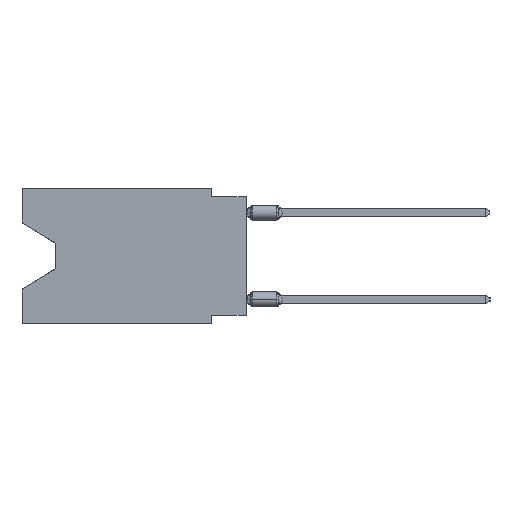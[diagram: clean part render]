
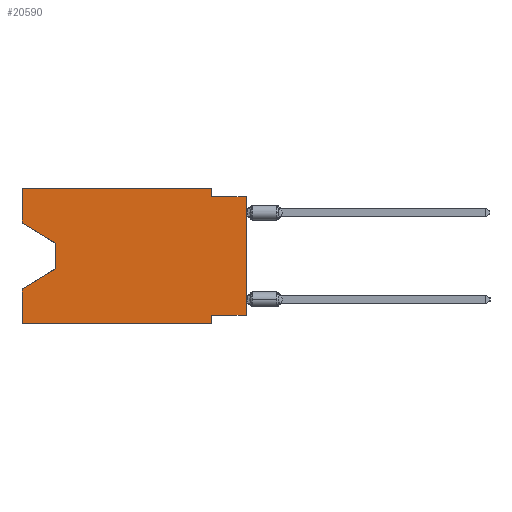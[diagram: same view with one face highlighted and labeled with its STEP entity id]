
A CAD part, left-side view. The second image highlights one B-rep face of the part: STEP entity #20590.
In plain terms, the highlighted planar face has unit normal (-1, 0, 0).
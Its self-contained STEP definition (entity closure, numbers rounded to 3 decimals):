
#54 = ORIENTED_EDGE ( 'NONE', *, *, #9145, .F. ) ;
#492 = AXIS2_PLACEMENT_3D ( 'NONE', #55331, #2793, #37650 ) ;
#593 = CARTESIAN_POINT ( 'NONE',  ( 0., 16.383, 0. ) ) ;
#1018 = EDGE_LOOP ( 'NONE', ( #4741, #35743, #3270, #43502, #29991, #54, #26393, #41804, #6170, #9267, #16644, #18646 ) ) ;
#1906 = VECTOR ( 'NONE', #36949, 1000. ) ;
#2367 = LINE ( 'NONE', #6391, #1906 ) ;
#2661 = EDGE_CURVE ( 'NONE', #33258, #40335, #24436, .T. ) ;
#2711 = CARTESIAN_POINT ( 'NONE',  ( 0., 16.383, 0. ) ) ;
#2793 = DIRECTION ( 'NONE',  ( 1., 0., 0. ) ) ;
#2820 = LINE ( 'NONE', #47371, #49563 ) ;
#3062 = EDGE_CURVE ( 'NONE', #53417, #13756, #2367, .T. ) ;
#3233 = VECTOR ( 'NONE', #11815, 1000. ) ;
#3270 = ORIENTED_EDGE ( 'NONE', *, *, #39068, .T. ) ;
#3426 = EDGE_CURVE ( 'NONE', #18041, #45222, #9479, .T. ) ;
#3548 = EDGE_CURVE ( 'NONE', #38810, #24985, #23474, .T. ) ;
#3928 = CARTESIAN_POINT ( 'NONE',  ( 0., 2.54, 0. ) ) ;
#4708 = CARTESIAN_POINT ( 'NONE',  ( 0., 13.97, -4.013 ) ) ;
#4741 = ORIENTED_EDGE ( 'NONE', *, *, #3548, .T. ) ;
#5100 = CARTESIAN_POINT ( 'NONE',  ( 0., 2.54, -9.906 ) ) ;
#6170 = ORIENTED_EDGE ( 'NONE', *, *, #18437, .F. ) ;
#6234 = CARTESIAN_POINT ( 'NONE',  ( 0., 13.97, -4.013 ) ) ;
#6391 = CARTESIAN_POINT ( 'NONE',  ( 0., 16.383, 0. ) ) ;
#6787 = VERTEX_POINT ( 'NONE', #23119 ) ;
#7640 = LINE ( 'NONE', #3928, #50952 ) ;
#9145 = EDGE_CURVE ( 'NONE', #18328, #13405, #28743, .T. ) ;
#9267 = ORIENTED_EDGE ( 'NONE', *, *, #42584, .F. ) ;
#9479 = LINE ( 'NONE', #26908, #35715 ) ;
#10612 = CARTESIAN_POINT ( 'NONE',  ( 0., 16.383, -2.546 ) ) ;
#10644 = CARTESIAN_POINT ( 'NONE',  ( 0., 2.54, 0. ) ) ;
#10819 = LINE ( 'NONE', #37380, #25836 ) ;
#11815 = DIRECTION ( 'NONE',  ( 0., 0.855, -0.519 ) ) ;
#12222 = FACE_OUTER_BOUND ( 'NONE', #1018, .T. ) ;
#12529 = EDGE_CURVE ( 'NONE', #53417, #13405, #22379, .T. ) ;
#12964 = CARTESIAN_POINT ( 'NONE',  ( 0., 16.383, -9.906 ) ) ;
#13405 = VERTEX_POINT ( 'NONE', #5100 ) ;
#13478 = EDGE_CURVE ( 'NONE', #24985, #6787, #27385, .T. ) ;
#13518 = DIRECTION ( 'NONE',  ( 0., -1., 0. ) ) ;
#13756 = VERTEX_POINT ( 'NONE', #19018 ) ;
#14717 = VECTOR ( 'NONE', #40891, 1000. ) ;
#16524 = VECTOR ( 'NONE', #36237, 1000. ) ;
#16644 = ORIENTED_EDGE ( 'NONE', *, *, #2661, .F. ) ;
#17366 = VECTOR ( 'NONE', #20144, 1000. ) ;
#18041 = VERTEX_POINT ( 'NONE', #33754 ) ;
#18328 = VERTEX_POINT ( 'NONE', #49402 ) ;
#18437 = EDGE_CURVE ( 'NONE', #20125, #45222, #2820, .T. ) ;
#18609 = CARTESIAN_POINT ( 'NONE',  ( 0., 2.54, -0.635 ) ) ;
#18646 = ORIENTED_EDGE ( 'NONE', *, *, #19426, .F. ) ;
#19018 = CARTESIAN_POINT ( 'NONE',  ( 0., 16.383, -7.36 ) ) ;
#19426 = EDGE_CURVE ( 'NONE', #38810, #33258, #48273, .T. ) ;
#20125 = VERTEX_POINT ( 'NONE', #18609 ) ;
#20144 = DIRECTION ( 'NONE',  ( 0., -1., 0. ) ) ;
#20590 = ADVANCED_FACE ( 'NONE', ( #12222 ), #41646, .F. ) ;
#22379 = LINE ( 'NONE', #12964, #37397 ) ;
#23119 = CARTESIAN_POINT ( 'NONE',  ( 0., 13.97, -5.893 ) ) ;
#23408 = DIRECTION ( 'NONE',  ( 0., 1., 0. ) ) ;
#23474 = LINE ( 'NONE', #10612, #14717 ) ;
#23980 = CARTESIAN_POINT ( 'NONE',  ( 0., 16.383, 0. ) ) ;
#24230 = CARTESIAN_POINT ( 'NONE',  ( 0., 0., -0.635 ) ) ;
#24436 = LINE ( 'NONE', #2711, #17366 ) ;
#24985 = VERTEX_POINT ( 'NONE', #4708 ) ;
#25836 = VECTOR ( 'NONE', #23408, 1000. ) ;
#26393 = ORIENTED_EDGE ( 'NONE', *, *, #36709, .F. ) ;
#26908 = CARTESIAN_POINT ( 'NONE',  ( 0., 0., 0. ) ) ;
#27385 = LINE ( 'NONE', #6234, #16524 ) ;
#28743 = LINE ( 'NONE', #46162, #53382 ) ;
#29991 = ORIENTED_EDGE ( 'NONE', *, *, #12529, .T. ) ;
#31446 = DIRECTION ( 'NONE',  ( 0., 0., 1. ) ) ;
#33258 = VERTEX_POINT ( 'NONE', #23980 ) ;
#33754 = CARTESIAN_POINT ( 'NONE',  ( 0., 0., -9.271 ) ) ;
#33968 = DIRECTION ( 'NONE',  ( 0., -1., 0. ) ) ;
#34199 = DIRECTION ( 'NONE',  ( 0., 0., -1. ) ) ;
#35066 = VECTOR ( 'NONE', #31446, 1000. ) ;
#35715 = VECTOR ( 'NONE', #36886, 1000. ) ;
#35743 = ORIENTED_EDGE ( 'NONE', *, *, #13478, .T. ) ;
#36237 = DIRECTION ( 'NONE',  ( 0., 0., -1. ) ) ;
#36709 = EDGE_CURVE ( 'NONE', #18041, #18328, #10819, .T. ) ;
#36886 = DIRECTION ( 'NONE',  ( 0., 0., 1. ) ) ;
#36949 = DIRECTION ( 'NONE',  ( 0., 0., 1. ) ) ;
#37380 = CARTESIAN_POINT ( 'NONE',  ( 0., 0., -9.271 ) ) ;
#37397 = VECTOR ( 'NONE', #13518, 1000. ) ;
#37650 = DIRECTION ( 'NONE',  ( 0., 0., -1. ) ) ;
#37815 = LINE ( 'NONE', #50940, #3233 ) ;
#38810 = VERTEX_POINT ( 'NONE', #46092 ) ;
#39068 = EDGE_CURVE ( 'NONE', #6787, #13756, #37815, .T. ) ;
#40335 = VERTEX_POINT ( 'NONE', #10644 ) ;
#40891 = DIRECTION ( 'NONE',  ( 0., -0.855, -0.519 ) ) ;
#41646 = PLANE ( 'NONE',  #492 ) ;
#41804 = ORIENTED_EDGE ( 'NONE', *, *, #3426, .T. ) ;
#41883 = DIRECTION ( 'NONE',  ( 0., 0., -1. ) ) ;
#42584 = EDGE_CURVE ( 'NONE', #40335, #20125, #7640, .T. ) ;
#43502 = ORIENTED_EDGE ( 'NONE', *, *, #3062, .F. ) ;
#45222 = VERTEX_POINT ( 'NONE', #24230 ) ;
#46092 = CARTESIAN_POINT ( 'NONE',  ( 0., 16.383, -2.546 ) ) ;
#46162 = CARTESIAN_POINT ( 'NONE',  ( 0., 2.54, -9.906 ) ) ;
#47371 = CARTESIAN_POINT ( 'NONE',  ( 0., 0., -0.635 ) ) ;
#47603 = CARTESIAN_POINT ( 'NONE',  ( 0., 16.383, -9.906 ) ) ;
#48273 = LINE ( 'NONE', #593, #35066 ) ;
#49402 = CARTESIAN_POINT ( 'NONE',  ( 0., 2.54, -9.271 ) ) ;
#49563 = VECTOR ( 'NONE', #33968, 1000. ) ;
#50940 = CARTESIAN_POINT ( 'NONE',  ( 0., 13.97, -5.893 ) ) ;
#50952 = VECTOR ( 'NONE', #34199, 1000. ) ;
#53382 = VECTOR ( 'NONE', #41883, 1000. ) ;
#53417 = VERTEX_POINT ( 'NONE', #47603 ) ;
#55331 = CARTESIAN_POINT ( 'NONE',  ( 0., 16.383, 0. ) ) ;
